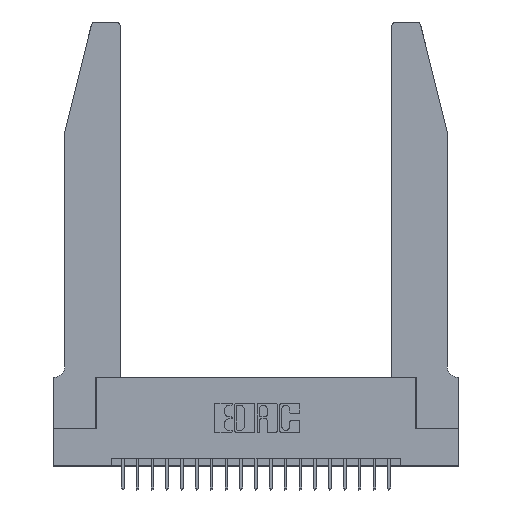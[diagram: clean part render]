
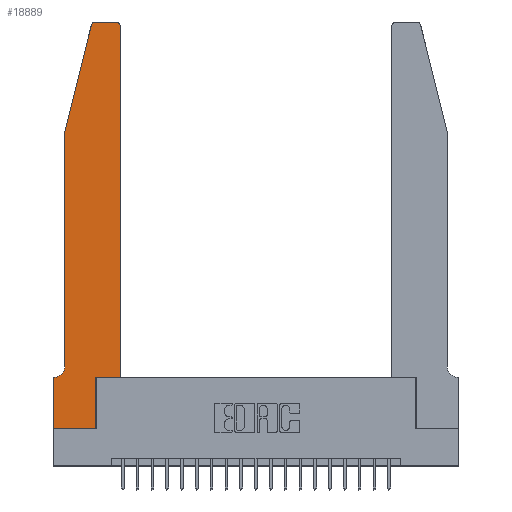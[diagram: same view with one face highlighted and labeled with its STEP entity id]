
A CAD part, top view. The second image highlights one B-rep face of the part: STEP entity #18889.
In plain terms, the highlighted planar face has unit normal (0, 0, 1).
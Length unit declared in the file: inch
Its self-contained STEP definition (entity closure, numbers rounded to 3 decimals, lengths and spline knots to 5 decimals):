
#48 = DIRECTION ( 'NONE',  ( 0., 1., 0. ) ) ;
#278 = DIRECTION ( 'NONE',  ( -1., 0., 0. ) ) ;
#301 = CARTESIAN_POINT ( 'NONE',  ( 0.2865, 0.35, 0.37 ) ) ;
#672 = VERTEX_POINT ( 'NONE', #12549 ) ;
#728 = DIRECTION ( 'NONE',  ( 0., 0., 1. ) ) ;
#747 = DIRECTION ( 'NONE',  ( 0., -1., 0. ) ) ;
#816 = DIRECTION ( 'NONE',  ( -1., 0., 0. ) ) ;
#936 = DIRECTION ( 'NONE',  ( -1., 0., 0. ) ) ;
#1306 = CIRCLE ( 'NONE', #17637, 0.03 ) ;
#1419 = AXIS2_PLACEMENT_3D ( 'NONE', #13364, #2705, #15096 ) ;
#2286 = VERTEX_POINT ( 'NONE', #5665 ) ;
#2314 = VECTOR ( 'NONE', #17077, 39.37008 ) ;
#2618 = CARTESIAN_POINT ( 'NONE',  ( 0., 0., 0.37 ) ) ;
#2705 = DIRECTION ( 'NONE',  ( 0., 0., 1. ) ) ;
#2838 = VERTEX_POINT ( 'NONE', #8776 ) ;
#3212 = ORIENTED_EDGE ( 'NONE', *, *, #9385, .T. ) ;
#3288 = EDGE_CURVE ( 'NONE', #16334, #2838, #19502, .T. ) ;
#3799 = CARTESIAN_POINT ( 'NONE',  ( 0.4505, 0.35, 0.37 ) ) ;
#3997 = EDGE_CURVE ( 'NONE', #14277, #18408, #17368, .T. ) ;
#4461 = CARTESIAN_POINT ( 'NONE',  ( 0., 0.35, 0.37 ) ) ;
#4520 = DIRECTION ( 'NONE',  ( 1., 0., 0. ) ) ;
#4634 = ORIENTED_EDGE ( 'NONE', *, *, #13045, .T. ) ;
#4867 = ORIENTED_EDGE ( 'NONE', *, *, #3997, .T. ) ;
#5611 = CARTESIAN_POINT ( 'NONE',  ( 0., 0.35, 0.37 ) ) ;
#5665 = CARTESIAN_POINT ( 'NONE',  ( 0.2865, 0., 0.37 ) ) ;
#5802 = AXIS2_PLACEMENT_3D ( 'NONE', #4461, #728, #13297 ) ;
#6253 = VECTOR ( 'NONE', #747, 39.37008 ) ;
#6677 = CARTESIAN_POINT ( 'NONE',  ( 0.0755, 2., 0.37 ) ) ;
#6999 = ORIENTED_EDGE ( 'NONE', *, *, #20826, .T. ) ;
#7407 = CIRCLE ( 'NONE', #18842, 0.07 ) ;
#7499 = LINE ( 'NONE', #3799, #10497 ) ;
#7589 = EDGE_CURVE ( 'NONE', #19010, #20322, #22566, .T. ) ;
#7685 = CARTESIAN_POINT ( 'NONE',  ( 0.0755, 2., 0.37 ) ) ;
#7894 = VECTOR ( 'NONE', #4520, 39.37008 ) ;
#8069 = VERTEX_POINT ( 'NONE', #20706 ) ;
#8078 = PLANE ( 'NONE',  #5802 ) ;
#8334 = ORIENTED_EDGE ( 'NONE', *, *, #19136, .T. ) ;
#8451 = VERTEX_POINT ( 'NONE', #11833 ) ;
#8776 = CARTESIAN_POINT ( 'NONE',  ( 0.0755, 0.42, 0.37 ) ) ;
#8902 = CARTESIAN_POINT ( 'NONE',  ( 0.2865, 0.35, 0.37 ) ) ;
#8984 = ORIENTED_EDGE ( 'NONE', *, *, #22198, .T. ) ;
#9194 = DIRECTION ( 'NONE',  ( 0., 0., 1. ) ) ;
#9385 = EDGE_CURVE ( 'NONE', #672, #8451, #1306, .T. ) ;
#9935 = CARTESIAN_POINT ( 'NONE',  ( 0., 0., 0.37 ) ) ;
#10230 = EDGE_CURVE ( 'NONE', #16246, #2286, #12502, .T. ) ;
#10497 = VECTOR ( 'NONE', #48, 39.37008 ) ;
#10575 = CARTESIAN_POINT ( 'NONE',  ( 0.284, 2.75, 0.37 ) ) ;
#11159 = DIRECTION ( 'NONE',  ( 0., 1., 0. ) ) ;
#11274 = VECTOR ( 'NONE', #11159, 39.37008 ) ;
#11643 = DIRECTION ( 'NONE',  ( 0., 0., -1. ) ) ;
#11833 = CARTESIAN_POINT ( 'NONE',  ( 0.4205, 2.75, 0.37 ) ) ;
#12096 = VECTOR ( 'NONE', #278, 39.37008 ) ;
#12389 = ORIENTED_EDGE ( 'NONE', *, *, #3288, .T. ) ;
#12502 = LINE ( 'NONE', #2618, #7894 ) ;
#12549 = CARTESIAN_POINT ( 'NONE',  ( 0.4505, 2.72, 0.37 ) ) ;
#12629 = CARTESIAN_POINT ( 'NONE',  ( 0., 0., 0.37 ) ) ;
#12878 = CARTESIAN_POINT ( 'NONE',  ( 0.2605, 2.75, 0.37 ) ) ;
#13045 = EDGE_CURVE ( 'NONE', #18408, #16334, #15885, .T. ) ;
#13226 = VERTEX_POINT ( 'NONE', #8902 ) ;
#13297 = DIRECTION ( 'NONE',  ( 1., 0., 0. ) ) ;
#13364 = CARTESIAN_POINT ( 'NONE',  ( 0.284, 2.72, 0.37 ) ) ;
#13442 = LINE ( 'NONE', #9935, #22045 ) ;
#13479 = ORIENTED_EDGE ( 'NONE', *, *, #14613, .T. ) ;
#14277 = VERTEX_POINT ( 'NONE', #10575 ) ;
#14556 = LINE ( 'NONE', #15966, #15135 ) ;
#14613 = EDGE_CURVE ( 'NONE', #2838, #19010, #7407, .T. ) ;
#15096 = DIRECTION ( 'NONE',  ( 1., 0., 0. ) ) ;
#15129 = ORIENTED_EDGE ( 'NONE', *, *, #22354, .T. ) ;
#15135 = VECTOR ( 'NONE', #17692, 39.37008 ) ;
#15884 = LINE ( 'NONE', #301, #11274 ) ;
#15885 = LINE ( 'NONE', #6677, #2314 ) ;
#15966 = CARTESIAN_POINT ( 'NONE',  ( 0.4505, 0.35, 0.37 ) ) ;
#16207 = ORIENTED_EDGE ( 'NONE', *, *, #10230, .T. ) ;
#16246 = VERTEX_POINT ( 'NONE', #12629 ) ;
#16334 = VERTEX_POINT ( 'NONE', #7685 ) ;
#17077 = DIRECTION ( 'NONE',  ( -0.239, -0.971, 0. ) ) ;
#17368 = CIRCLE ( 'NONE', #1419, 0.03 ) ;
#17637 = AXIS2_PLACEMENT_3D ( 'NONE', #19519, #9194, #21243 ) ;
#17692 = DIRECTION ( 'NONE',  ( 1., 0., 0. ) ) ;
#18009 = VECTOR ( 'NONE', #936, 39.37008 ) ;
#18408 = VERTEX_POINT ( 'NONE', #22330 ) ;
#18520 = DIRECTION ( 'NONE',  ( 0., -1., 0. ) ) ;
#18842 = AXIS2_PLACEMENT_3D ( 'NONE', #21935, #11643, #816 ) ;
#18889 = ADVANCED_FACE ( 'NONE', ( #19919 ), #8078, .T. ) ;
#18891 = ORIENTED_EDGE ( 'NONE', *, *, #19763, .T. ) ;
#19010 = VERTEX_POINT ( 'NONE', #20629 ) ;
#19136 = EDGE_CURVE ( 'NONE', #8069, #672, #7499, .T. ) ;
#19502 = LINE ( 'NONE', #21880, #6253 ) ;
#19519 = CARTESIAN_POINT ( 'NONE',  ( 0.4205, 2.72, 0.37 ) ) ;
#19763 = EDGE_CURVE ( 'NONE', #2286, #13226, #15884, .T. ) ;
#19919 = FACE_OUTER_BOUND ( 'NONE', #20162, .T. ) ;
#20162 = EDGE_LOOP ( 'NONE', ( #8984, #4867, #4634, #12389, #13479, #21263, #15129, #16207, #18891, #6999, #8334, #3212 ) ) ;
#20322 = VERTEX_POINT ( 'NONE', #5611 ) ;
#20629 = CARTESIAN_POINT ( 'NONE',  ( 0.0055, 0.35, 0.37 ) ) ;
#20706 = CARTESIAN_POINT ( 'NONE',  ( 0.4505, 0.35, 0.37 ) ) ;
#20826 = EDGE_CURVE ( 'NONE', #13226, #8069, #14556, .T. ) ;
#21222 = LINE ( 'NONE', #12878, #12096 ) ;
#21243 = DIRECTION ( 'NONE',  ( 1., 0., 0. ) ) ;
#21263 = ORIENTED_EDGE ( 'NONE', *, *, #7589, .T. ) ;
#21880 = CARTESIAN_POINT ( 'NONE',  ( 0.0755, 2., 0.37 ) ) ;
#21935 = CARTESIAN_POINT ( 'NONE',  ( 0.0055, 0.42, 0.37 ) ) ;
#22042 = CARTESIAN_POINT ( 'NONE',  ( 0.0755, 0.35, 0.37 ) ) ;
#22045 = VECTOR ( 'NONE', #18520, 39.37008 ) ;
#22198 = EDGE_CURVE ( 'NONE', #8451, #14277, #21222, .T. ) ;
#22330 = CARTESIAN_POINT ( 'NONE',  ( 0.25487, 2.72718, 0.37 ) ) ;
#22354 = EDGE_CURVE ( 'NONE', #20322, #16246, #13442, .T. ) ;
#22566 = LINE ( 'NONE', #22042, #18009 ) ;
